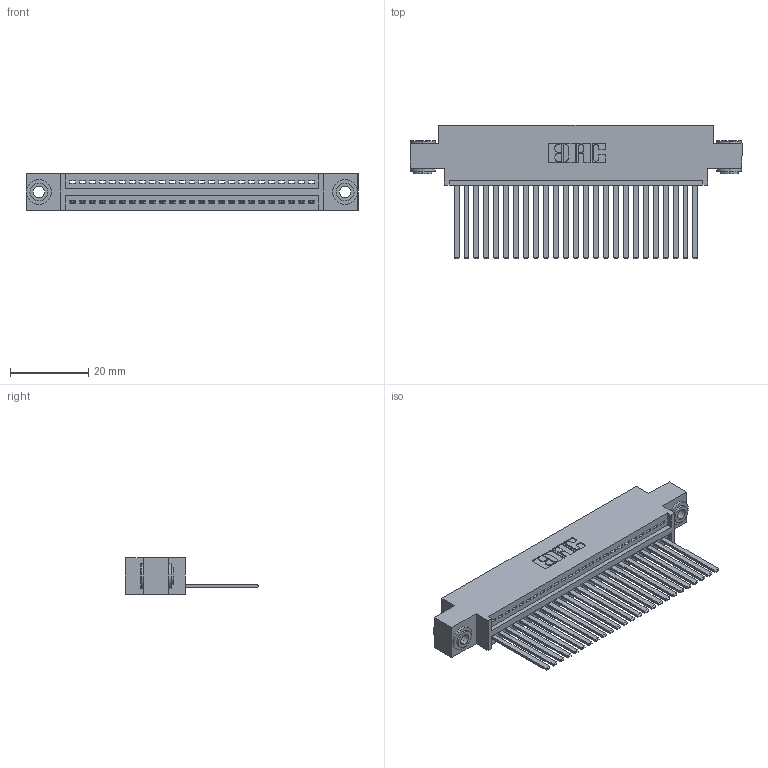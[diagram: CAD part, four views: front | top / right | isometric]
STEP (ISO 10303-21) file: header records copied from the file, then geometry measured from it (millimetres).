
FILE_DESCRIPTION (( 'STEP AP203' ), '1' );
FILE_NAME ('345-025-544-603.STEP', '2019-10-05T07:41:57', ( '' ), ( '' ), 'SwSTEP 2.0', 'SolidWorks 2016', '' );
FILE_SCHEMA (( 'CONFIG_CONTROL_DESIGN' ));
Length unit declared in the file: inch
Products named in the file (4): 345-025-544-603; 345-292-001_345-293-144; 345-250-002_345-250-002-102; 345 Part_0.170 Offset - 0.156 Dia-TH
Assembly tree (28 placements, depth 2):
  345-025-544-603
    345 Part_0.170 Offset - 0.156 Dia-TH
    345-292-001_345-293-144  x25
    345-250-002_345-250-002-102  x2
Bounding box: 84.71 x 33.96 x 9.4 mm (x, y, z)
Volume: 8102 mm3; surface area: 11746.1 mm2
Topology: 28 solids, 28 shells, 1468 faces, 4379 edges, 2882 vertices
Faces by surface type: plane 994, cylinder 466, cone 8
Entity records: 21702 total; most frequent: CARTESIAN_POINT 3738, ORIENTED_EDGE 3690, DIRECTION 3317, EDGE_CURVE 1845, LINE 1593, VECTOR 1593, VERTEX_POINT 1226, AXIS2_PLACEMENT_3D 862
